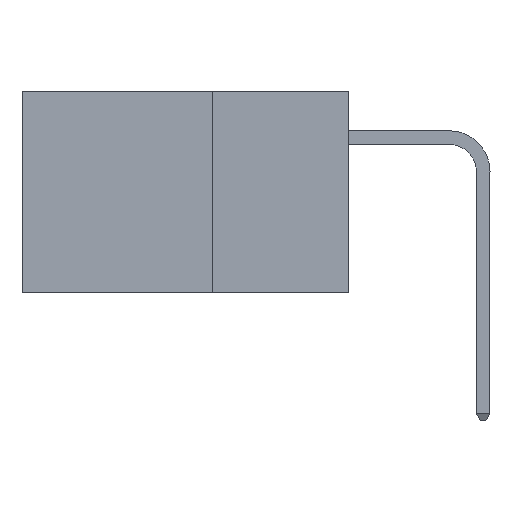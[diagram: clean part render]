
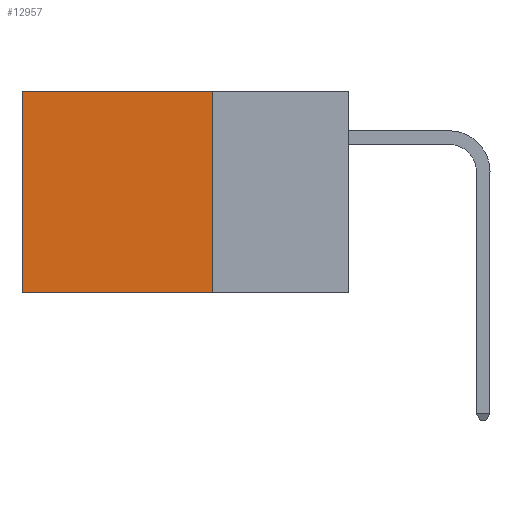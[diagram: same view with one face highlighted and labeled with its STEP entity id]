
A CAD part, left-side view. The second image highlights one B-rep face of the part: STEP entity #12957.
In plain terms, the highlighted planar face has unit normal (-1, 0, 0).
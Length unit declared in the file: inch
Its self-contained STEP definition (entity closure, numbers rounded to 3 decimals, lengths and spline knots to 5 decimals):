
#9 = ORIENTED_EDGE ( 'NONE', *, *, #2733, .T. ) ;
#124 = DIRECTION ( 'NONE',  ( 0., 1., 0. ) ) ;
#1212 = DIRECTION ( 'NONE',  ( 0., 0., -1. ) ) ;
#1579 = VERTEX_POINT ( 'NONE', #10036 ) ;
#1767 = CARTESIAN_POINT ( 'NONE',  ( 0.2875, 0.25, -0.37 ) ) ;
#1898 = CARTESIAN_POINT ( 'NONE',  ( 0.2875, 0.25, 0. ) ) ;
#2213 = VECTOR ( 'NONE', #9884, 39.37008 ) ;
#2234 = LINE ( 'NONE', #10837, #2909 ) ;
#2601 = DIRECTION ( 'NONE',  ( 0., 1., 0. ) ) ;
#2733 = EDGE_CURVE ( 'NONE', #1579, #12156, #4388, .T. ) ;
#2909 = VECTOR ( 'NONE', #1212, 39.37008 ) ;
#3357 = VECTOR ( 'NONE', #2601, 39.37008 ) ;
#3386 = CARTESIAN_POINT ( 'NONE',  ( 0.2875, 0.6, 0. ) ) ;
#3794 = ORIENTED_EDGE ( 'NONE', *, *, #5478, .T. ) ;
#3814 = CARTESIAN_POINT ( 'NONE',  ( 0.2875, 0.6, -0.37 ) ) ;
#4026 = EDGE_CURVE ( 'NONE', #9065, #12156, #11664, .T. ) ;
#4088 = DIRECTION ( 'NONE',  ( 1., 0., 0. ) ) ;
#4198 = CARTESIAN_POINT ( 'NONE',  ( 0.2875, 0.25, 0. ) ) ;
#4388 = LINE ( 'NONE', #3386, #2213 ) ;
#5196 = DIRECTION ( 'NONE',  ( 0., 0., -1. ) ) ;
#5478 = EDGE_CURVE ( 'NONE', #8387, #1579, #11612, .T. ) ;
#6287 = CARTESIAN_POINT ( 'NONE',  ( 0.2875, 0.25, 0. ) ) ;
#7148 = VECTOR ( 'NONE', #124, 39.37008 ) ;
#7987 = CARTESIAN_POINT ( 'NONE',  ( 0.2875, 0.25, -0.37 ) ) ;
#8387 = VERTEX_POINT ( 'NONE', #4198 ) ;
#8509 = AXIS2_PLACEMENT_3D ( 'NONE', #1898, #4088, #5196 ) ;
#8579 = ORIENTED_EDGE ( 'NONE', *, *, #4026, .F. ) ;
#8907 = ORIENTED_EDGE ( 'NONE', *, *, #11777, .F. ) ;
#9065 = VERTEX_POINT ( 'NONE', #1767 ) ;
#9884 = DIRECTION ( 'NONE',  ( 0., 0., -1. ) ) ;
#10036 = CARTESIAN_POINT ( 'NONE',  ( 0.2875, 0.6, 0. ) ) ;
#10837 = CARTESIAN_POINT ( 'NONE',  ( 0.2875, 0.25, 0. ) ) ;
#11612 = LINE ( 'NONE', #6287, #7148 ) ;
#11664 = LINE ( 'NONE', #7987, #3357 ) ;
#11777 = EDGE_CURVE ( 'NONE', #8387, #9065, #2234, .T. ) ;
#12156 = VERTEX_POINT ( 'NONE', #3814 ) ;
#12957 = ADVANCED_FACE ( 'NONE', ( #13627 ), #13633, .F. ) ;
#13476 = EDGE_LOOP ( 'NONE', ( #9, #8579, #8907, #3794 ) ) ;
#13627 = FACE_OUTER_BOUND ( 'NONE', #13476, .T. ) ;
#13633 = PLANE ( 'NONE',  #8509 ) ;
